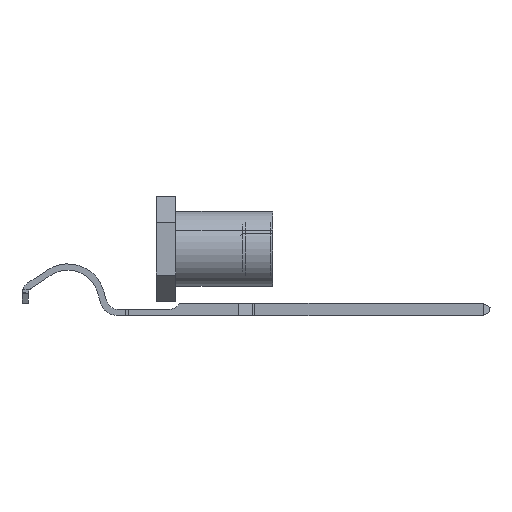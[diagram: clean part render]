
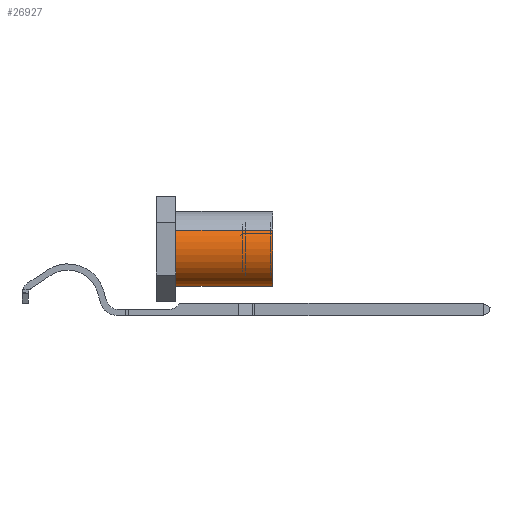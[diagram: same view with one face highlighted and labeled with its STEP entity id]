
A CAD part, left-side view. The second image highlights one B-rep face of the part: STEP entity #26927.
In plain terms, the highlighted cylindrical face has radius 1.968 mm (diameter 3.937 mm), a partial arc.
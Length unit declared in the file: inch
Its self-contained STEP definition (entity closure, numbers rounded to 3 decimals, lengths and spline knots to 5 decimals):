
#552 = CIRCLE ( 'NONE', #22359, 0.0775 ) ;
#1737 = CARTESIAN_POINT ( 'NONE',  ( 0., 0.24, 0.0775 ) ) ;
#2114 = AXIS2_PLACEMENT_3D ( 'NONE', #19627, #6374, #21860 ) ;
#2471 = DIRECTION ( 'NONE',  ( 0., 0., -1. ) ) ;
#5695 = CIRCLE ( 'NONE', #2114, 0.0775 ) ;
#6031 = VERTEX_POINT ( 'NONE', #26635 ) ;
#6213 = DIRECTION ( 'NONE',  ( 0., -1., 0. ) ) ;
#6266 = DIRECTION ( 'NONE',  ( 0., -1., 0. ) ) ;
#6374 = DIRECTION ( 'NONE',  ( 0., 1., 0. ) ) ;
#7685 = DIRECTION ( 'NONE',  ( 0., 1., 0. ) ) ;
#9948 = VERTEX_POINT ( 'NONE', #17136 ) ;
#10276 = VECTOR ( 'NONE', #6266, 39.37008 ) ;
#10489 = EDGE_LOOP ( 'NONE', ( #21055, #25863, #13024, #23327 ) ) ;
#10974 = LINE ( 'NONE', #24013, #10276 ) ;
#11375 = CARTESIAN_POINT ( 'NONE',  ( 0., 0.24, 0. ) ) ;
#11846 = EDGE_CURVE ( 'NONE', #13443, #14922, #10974, .T. ) ;
#11884 = FACE_OUTER_BOUND ( 'NONE', #10489, .T. ) ;
#12279 = EDGE_CURVE ( 'NONE', #14922, #9948, #552, .T. ) ;
#13024 = ORIENTED_EDGE ( 'NONE', *, *, #11846, .T. ) ;
#13443 = VERTEX_POINT ( 'NONE', #13887 ) ;
#13887 = CARTESIAN_POINT ( 'NONE',  ( 0., 0.24, -0.0775 ) ) ;
#14922 = VERTEX_POINT ( 'NONE', #25980 ) ;
#15126 = LINE ( 'NONE', #1737, #26996 ) ;
#17055 = CYLINDRICAL_SURFACE ( 'NONE', #20725, 0.0775 ) ;
#17136 = CARTESIAN_POINT ( 'NONE',  ( 0., 0.04, 0.0775 ) ) ;
#19326 = EDGE_CURVE ( 'NONE', #6031, #9948, #15126, .T. ) ;
#19627 = CARTESIAN_POINT ( 'NONE',  ( 0., 0.24, 0. ) ) ;
#20725 = AXIS2_PLACEMENT_3D ( 'NONE', #11375, #24683, #2471 ) ;
#20936 = CARTESIAN_POINT ( 'NONE',  ( 0., 0.04, 0. ) ) ;
#21055 = ORIENTED_EDGE ( 'NONE', *, *, #19326, .F. ) ;
#21860 = DIRECTION ( 'NONE',  ( 0., 0., 1. ) ) ;
#22359 = AXIS2_PLACEMENT_3D ( 'NONE', #20936, #7685, #23218 ) ;
#22729 = EDGE_CURVE ( 'NONE', #13443, #6031, #5695, .T. ) ;
#23218 = DIRECTION ( 'NONE',  ( 0., 0., 1. ) ) ;
#23327 = ORIENTED_EDGE ( 'NONE', *, *, #12279, .T. ) ;
#24013 = CARTESIAN_POINT ( 'NONE',  ( 0., 0.24, -0.0775 ) ) ;
#24683 = DIRECTION ( 'NONE',  ( 0., -1., 0. ) ) ;
#25863 = ORIENTED_EDGE ( 'NONE', *, *, #22729, .F. ) ;
#25980 = CARTESIAN_POINT ( 'NONE',  ( 0., 0.04, -0.0775 ) ) ;
#26635 = CARTESIAN_POINT ( 'NONE',  ( 0., 0.24, 0.0775 ) ) ;
#26927 = ADVANCED_FACE ( 'NONE', ( #11884 ), #17055, .T. ) ;
#26996 = VECTOR ( 'NONE', #6213, 39.37008 ) ;
